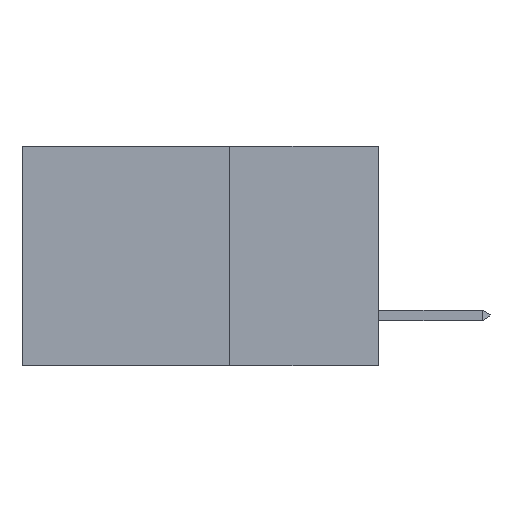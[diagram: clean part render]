
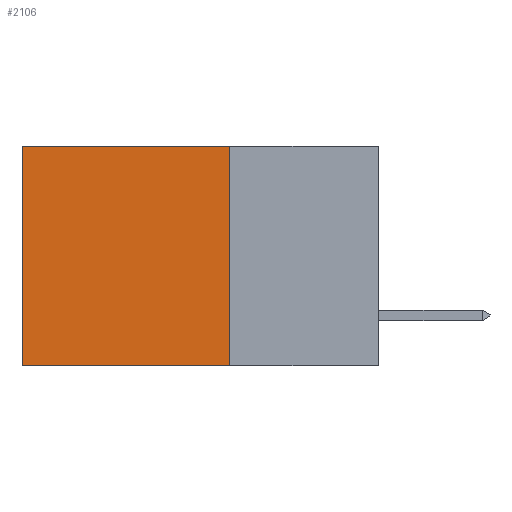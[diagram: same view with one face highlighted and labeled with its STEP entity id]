
A CAD part, left-side view. The second image highlights one B-rep face of the part: STEP entity #2106.
In plain terms, the highlighted planar face has unit normal (-1, 0, 0).
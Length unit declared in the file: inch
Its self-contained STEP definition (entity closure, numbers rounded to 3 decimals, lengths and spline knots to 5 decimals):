
#161 = CARTESIAN_POINT ( 'NONE',  ( 0.2615, 0.25, -0.37 ) ) ;
#185 = DIRECTION ( 'NONE',  ( 0., 0., -1. ) ) ;
#285 = ORIENTED_EDGE ( 'NONE', *, *, #11216, .T. ) ;
#724 = ORIENTED_EDGE ( 'NONE', *, *, #8709, .T. ) ;
#756 = VERTEX_POINT ( 'NONE', #161 ) ;
#796 = VERTEX_POINT ( 'NONE', #7069 ) ;
#908 = DIRECTION ( 'NONE',  ( 0., 0., -1. ) ) ;
#1214 = VERTEX_POINT ( 'NONE', #3779 ) ;
#1424 = CARTESIAN_POINT ( 'NONE',  ( 0.2615, 0.25, -0.37 ) ) ;
#1550 = ORIENTED_EDGE ( 'NONE', *, *, #2896, .F. ) ;
#2106 = ADVANCED_FACE ( 'NONE', ( #6984 ), #10689, .F. ) ;
#2332 = DIRECTION ( 'NONE',  ( 1., 0., 0. ) ) ;
#2753 = VECTOR ( 'NONE', #185, 39.37008 ) ;
#2896 = EDGE_CURVE ( 'NONE', #756, #3973, #11684, .T. ) ;
#3779 = CARTESIAN_POINT ( 'NONE',  ( 0.2615, 0.6, 0. ) ) ;
#3973 = VERTEX_POINT ( 'NONE', #8720 ) ;
#4394 = VECTOR ( 'NONE', #10660, 39.37008 ) ;
#4542 = LINE ( 'NONE', #5622, #8493 ) ;
#5299 = EDGE_CURVE ( 'NONE', #796, #756, #7639, .T. ) ;
#5622 = CARTESIAN_POINT ( 'NONE',  ( 0.2615, 0.6, -0.37 ) ) ;
#5842 = LINE ( 'NONE', #8396, #7086 ) ;
#5965 = ORIENTED_EDGE ( 'NONE', *, *, #5299, .F. ) ;
#6071 = DIRECTION ( 'NONE',  ( 0., 0., -1. ) ) ;
#6518 = AXIS2_PLACEMENT_3D ( 'NONE', #1424, #2332, #6071 ) ;
#6811 = DIRECTION ( 'NONE',  ( 0., 1., 0. ) ) ;
#6984 = FACE_OUTER_BOUND ( 'NONE', #9756, .T. ) ;
#7069 = CARTESIAN_POINT ( 'NONE',  ( 0.2615, 0.25, 0. ) ) ;
#7086 = VECTOR ( 'NONE', #6811, 39.37008 ) ;
#7639 = LINE ( 'NONE', #10441, #2753 ) ;
#8396 = CARTESIAN_POINT ( 'NONE',  ( 0.2615, 0.25, 0. ) ) ;
#8493 = VECTOR ( 'NONE', #908, 39.37008 ) ;
#8709 = EDGE_CURVE ( 'NONE', #796, #1214, #5842, .T. ) ;
#8720 = CARTESIAN_POINT ( 'NONE',  ( 0.2615, 0.6, -0.37 ) ) ;
#9691 = CARTESIAN_POINT ( 'NONE',  ( 0.2615, 0.25, -0.37 ) ) ;
#9756 = EDGE_LOOP ( 'NONE', ( #285, #1550, #5965, #724 ) ) ;
#10441 = CARTESIAN_POINT ( 'NONE',  ( 0.2615, 0.25, -0.37 ) ) ;
#10660 = DIRECTION ( 'NONE',  ( 0., 1., 0. ) ) ;
#10689 = PLANE ( 'NONE',  #6518 ) ;
#11216 = EDGE_CURVE ( 'NONE', #1214, #3973, #4542, .T. ) ;
#11684 = LINE ( 'NONE', #9691, #4394 ) ;
